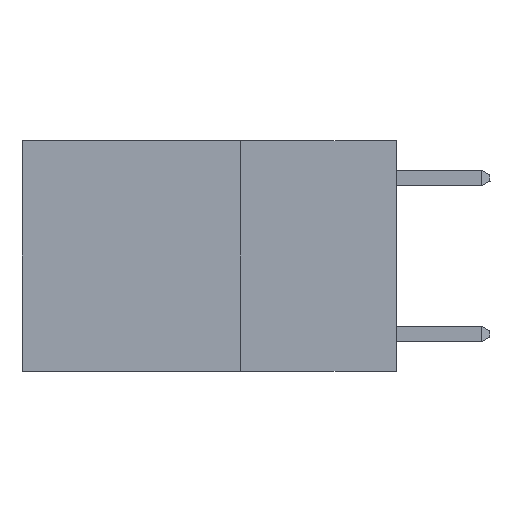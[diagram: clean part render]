
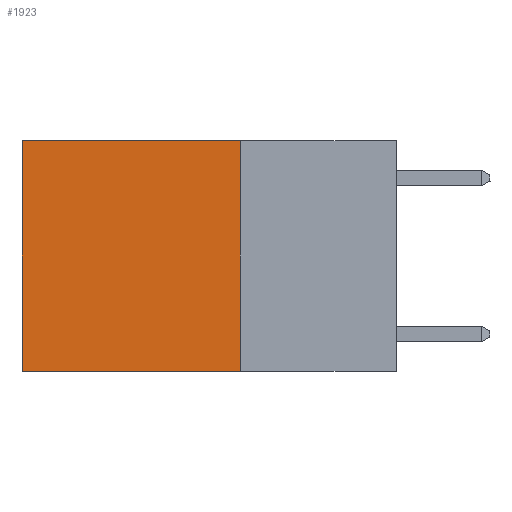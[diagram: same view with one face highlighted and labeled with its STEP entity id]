
A CAD part, left-side view. The second image highlights one B-rep face of the part: STEP entity #1923.
In plain terms, the highlighted planar face has unit normal (-1, 0, 0).
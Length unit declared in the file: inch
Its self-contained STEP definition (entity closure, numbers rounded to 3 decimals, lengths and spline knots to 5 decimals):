
#13 = DIRECTION ( 'NONE',  ( 0., 0., -1. ) ) ;
#704 = CARTESIAN_POINT ( 'NONE',  ( 0.2625, 0.25, 0. ) ) ;
#819 = DIRECTION ( 'NONE',  ( 0., 0., -1. ) ) ;
#823 = ORIENTED_EDGE ( 'NONE', *, *, #6432, .F. ) ;
#1121 = DIRECTION ( 'NONE',  ( 0., 1., 0. ) ) ;
#1247 = VECTOR ( 'NONE', #6822, 39.37008 ) ;
#1308 = CARTESIAN_POINT ( 'NONE',  ( 0.2625, 0.25, 0. ) ) ;
#1923 = ADVANCED_FACE ( 'NONE', ( #3596 ), #2552, .F. ) ;
#1930 = DIRECTION ( 'NONE',  ( 1., 0., 0. ) ) ;
#2245 = CARTESIAN_POINT ( 'NONE',  ( 0.2625, 0.25, 0. ) ) ;
#2396 = VERTEX_POINT ( 'NONE', #4034 ) ;
#2552 = PLANE ( 'NONE',  #7785 ) ;
#3058 = VECTOR ( 'NONE', #1121, 39.37008 ) ;
#3314 = VECTOR ( 'NONE', #13, 39.37008 ) ;
#3596 = FACE_OUTER_BOUND ( 'NONE', #5063, .T. ) ;
#3603 = CARTESIAN_POINT ( 'NONE',  ( 0.2625, 0.25, -0.37 ) ) ;
#3626 = LINE ( 'NONE', #2245, #1247 ) ;
#4034 = CARTESIAN_POINT ( 'NONE',  ( 0.2625, 0.6, 0. ) ) ;
#4159 = VERTEX_POINT ( 'NONE', #5450 ) ;
#4199 = ORIENTED_EDGE ( 'NONE', *, *, #6084, .F. ) ;
#4704 = LINE ( 'NONE', #7108, #3314 ) ;
#4818 = ORIENTED_EDGE ( 'NONE', *, *, #6826, .T. ) ;
#5063 = EDGE_LOOP ( 'NONE', ( #4818, #823, #4199, #6762 ) ) ;
#5450 = CARTESIAN_POINT ( 'NONE',  ( 0.2625, 0.6, -0.37 ) ) ;
#5494 = CARTESIAN_POINT ( 'NONE',  ( 0.2625, 0.6, 0. ) ) ;
#5733 = LINE ( 'NONE', #5494, #7561 ) ;
#6084 = EDGE_CURVE ( 'NONE', #6963, #6141, #4704, .T. ) ;
#6141 = VERTEX_POINT ( 'NONE', #7646 ) ;
#6432 = EDGE_CURVE ( 'NONE', #6141, #4159, #6906, .T. ) ;
#6762 = ORIENTED_EDGE ( 'NONE', *, *, #7202, .T. ) ;
#6822 = DIRECTION ( 'NONE',  ( 0., 1., 0. ) ) ;
#6826 = EDGE_CURVE ( 'NONE', #2396, #4159, #5733, .T. ) ;
#6883 = DIRECTION ( 'NONE',  ( 0., 0., -1. ) ) ;
#6906 = LINE ( 'NONE', #3603, #3058 ) ;
#6963 = VERTEX_POINT ( 'NONE', #1308 ) ;
#7108 = CARTESIAN_POINT ( 'NONE',  ( 0.2625, 0.25, 0. ) ) ;
#7202 = EDGE_CURVE ( 'NONE', #6963, #2396, #3626, .T. ) ;
#7561 = VECTOR ( 'NONE', #6883, 39.37008 ) ;
#7646 = CARTESIAN_POINT ( 'NONE',  ( 0.2625, 0.25, -0.37 ) ) ;
#7785 = AXIS2_PLACEMENT_3D ( 'NONE', #704, #1930, #819 ) ;
